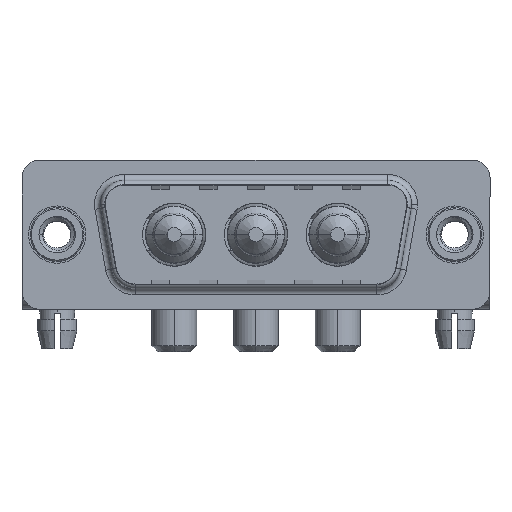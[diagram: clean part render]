
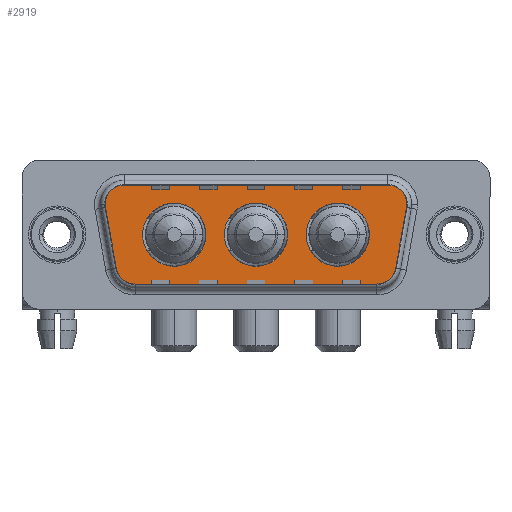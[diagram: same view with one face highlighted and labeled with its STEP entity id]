
A CAD part, top view. The second image highlights one B-rep face of the part: STEP entity #2919.
In plain terms, the highlighted planar face has unit normal (0, 0, 1).
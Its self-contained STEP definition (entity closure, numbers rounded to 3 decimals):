
#62 = CIRCLE ( 'NONE', #9373, 2. ) ;
#112 = DIRECTION ( 'NONE',  ( 0., 0., 1. ) ) ;
#334 = AXIS2_PLACEMENT_3D ( 'NONE', #9190, #4175, #4257 ) ;
#494 = VERTEX_POINT ( 'NONE', #16074 ) ;
#669 = ORIENTED_EDGE ( 'NONE', *, *, #7962, .T. ) ;
#758 = FACE_OUTER_BOUND ( 'NONE', #4294, .T. ) ;
#973 = VERTEX_POINT ( 'NONE', #8131 ) ;
#975 = DIRECTION ( 'NONE',  ( 0.174, -0.985, 0. ) ) ;
#1321 = CARTESIAN_POINT ( 'NONE',  ( 4.464, -3.247, 0. ) ) ;
#1376 = CIRCLE ( 'NONE', #2183, 2. ) ;
#1502 = EDGE_LOOP ( 'NONE', ( #6239, #13874 ) ) ;
#2003 = ORIENTED_EDGE ( 'NONE', *, *, #2544, .T. ) ;
#2026 = DIRECTION ( 'NONE',  ( 0., 0., 1. ) ) ;
#2038 = EDGE_CURVE ( 'NONE', #14971, #13674, #3644, .T. ) ;
#2063 = DIRECTION ( 'NONE',  ( 0., 0., 1. ) ) ;
#2183 = AXIS2_PLACEMENT_3D ( 'NONE', #11516, #112, #14067 ) ;
#2236 = ORIENTED_EDGE ( 'NONE', *, *, #15955, .T. ) ;
#2244 = CARTESIAN_POINT ( 'NONE',  ( 19.3, 0., 0. ) ) ;
#2288 = DIRECTION ( 'NONE',  ( -1., 0., 0. ) ) ;
#2383 = CIRCLE ( 'NONE', #10091, 2. ) ;
#2413 = CARTESIAN_POINT ( 'NONE',  ( 3.441, 2.553, 0. ) ) ;
#2451 = DIRECTION ( 'NONE',  ( 0., 0., 1. ) ) ;
#2472 = VERTEX_POINT ( 'NONE', #14736 ) ;
#2508 = CARTESIAN_POINT ( 'NONE',  ( 27.889, 4.9, 0. ) ) ;
#2544 = EDGE_CURVE ( 'NONE', #7589, #12192, #7376, .T. ) ;
#2668 = AXIS2_PLACEMENT_3D ( 'NONE', #5523, #10586, #3020 ) ;
#2671 = CARTESIAN_POINT ( 'NONE',  ( 6.434, -4.9, 0. ) ) ;
#2919 = ADVANCED_FACE ( 'NONE', ( #9772, #12248, #7093, #758 ), #3181, .T. ) ;
#3020 = DIRECTION ( 'NONE',  ( 1., 0., 0. ) ) ;
#3071 = ORIENTED_EDGE ( 'NONE', *, *, #7793, .T. ) ;
#3181 = PLANE ( 'NONE',  #11221 ) ;
#3267 = DIRECTION ( 'NONE',  ( 0., 0., 1. ) ) ;
#3330 = CARTESIAN_POINT ( 'NONE',  ( 7.15, 0., 0. ) ) ;
#3361 = CARTESIAN_POINT ( 'NONE',  ( 26.866, -4.9, 0. ) ) ;
#3372 = DIRECTION ( 'NONE',  ( -1., 0., 0. ) ) ;
#3630 = EDGE_CURVE ( 'NONE', #5560, #13367, #10240, .T. ) ;
#3644 = LINE ( 'NONE', #16088, #15944 ) ;
#3901 = CARTESIAN_POINT ( 'NONE',  ( 16.65, 0., 0. ) ) ;
#3973 = CIRCLE ( 'NONE', #14322, 2.65 ) ;
#4175 = DIRECTION ( 'NONE',  ( 0., 0., 1. ) ) ;
#4257 = DIRECTION ( 'NONE',  ( 1., 0., 0. ) ) ;
#4294 = EDGE_LOOP ( 'NONE', ( #5574, #669, #2236, #9229, #2003, #10066, #11195, #3071, #12345 ) ) ;
#4396 = CARTESIAN_POINT ( 'NONE',  ( 6.434, -2.9, 0. ) ) ;
#4527 = CIRCLE ( 'NONE', #9333, 2. ) ;
#4597 = CARTESIAN_POINT ( 'NONE',  ( 26.866, -2.9, 0. ) ) ;
#4657 = VERTEX_POINT ( 'NONE', #12388 ) ;
#4755 = CIRCLE ( 'NONE', #11416, 2.65 ) ;
#4865 = EDGE_CURVE ( 'NONE', #13472, #2472, #13199, .T. ) ;
#5523 = CARTESIAN_POINT ( 'NONE',  ( 16.65, 0., 0. ) ) ;
#5560 = VERTEX_POINT ( 'NONE', #10614 ) ;
#5574 = ORIENTED_EDGE ( 'NONE', *, *, #9288, .T. ) ;
#5813 = DIRECTION ( 'NONE',  ( 0., 0., 1. ) ) ;
#5927 = ORIENTED_EDGE ( 'NONE', *, *, #12511, .F. ) ;
#6073 = LINE ( 'NONE', #7316, #9551 ) ;
#6239 = ORIENTED_EDGE ( 'NONE', *, *, #7839, .F. ) ;
#6382 = DIRECTION ( 'NONE',  ( 0.174, 0.985, 0. ) ) ;
#6457 = CIRCLE ( 'NONE', #334, 2.65 ) ;
#6818 = ORIENTED_EDGE ( 'NONE', *, *, #16367, .F. ) ;
#6961 = VERTEX_POINT ( 'NONE', #14890 ) ;
#6987 = DIRECTION ( 'NONE',  ( 1., 0., 0. ) ) ;
#7093 = FACE_BOUND ( 'NONE', #1502, .T. ) ;
#7098 = DIRECTION ( 'NONE',  ( 0., 0., 1. ) ) ;
#7143 = DIRECTION ( 'NONE',  ( -1., 0., 0. ) ) ;
#7196 = DIRECTION ( 'NONE',  ( 0., 0., 1. ) ) ;
#7282 = CARTESIAN_POINT ( 'NONE',  ( 26.866, -2.9, 0. ) ) ;
#7316 = CARTESIAN_POINT ( 'NONE',  ( 29.859, 2.553, 0. ) ) ;
#7376 = LINE ( 'NONE', #16160, #10085 ) ;
#7571 = CARTESIAN_POINT ( 'NONE',  ( 28.836, -3.247, 0. ) ) ;
#7579 = DIRECTION ( 'NONE',  ( 0., 0., 1. ) ) ;
#7589 = VERTEX_POINT ( 'NONE', #2508 ) ;
#7793 = EDGE_CURVE ( 'NONE', #13674, #5560, #16162, .T. ) ;
#7839 = EDGE_CURVE ( 'NONE', #494, #14833, #8766, .T. ) ;
#7939 = EDGE_CURVE ( 'NONE', #6961, #10561, #4755, .T. ) ;
#7962 = EDGE_CURVE ( 'NONE', #13678, #4657, #6073, .T. ) ;
#7992 = CIRCLE ( 'NONE', #2668, 2.65 ) ;
#8085 = CARTESIAN_POINT ( 'NONE',  ( 9.8, 0., 0. ) ) ;
#8131 = CARTESIAN_POINT ( 'NONE',  ( 29.889, 2.9, 0. ) ) ;
#8205 = EDGE_CURVE ( 'NONE', #14833, #494, #3973, .T. ) ;
#8539 = EDGE_LOOP ( 'NONE', ( #15454, #6818 ) ) ;
#8766 = CIRCLE ( 'NONE', #10340, 2.65 ) ;
#8877 = ORIENTED_EDGE ( 'NONE', *, *, #7939, .F. ) ;
#9190 = CARTESIAN_POINT ( 'NONE',  ( 23.5, 0., 0. ) ) ;
#9229 = ORIENTED_EDGE ( 'NONE', *, *, #12209, .T. ) ;
#9256 = AXIS2_PLACEMENT_3D ( 'NONE', #3901, #7579, #15112 ) ;
#9288 = EDGE_CURVE ( 'NONE', #13367, #13678, #4527, .T. ) ;
#9333 = AXIS2_PLACEMENT_3D ( 'NONE', #7282, #7196, #9531 ) ;
#9373 = AXIS2_PLACEMENT_3D ( 'NONE', #10108, #2451, #12837 ) ;
#9531 = DIRECTION ( 'NONE',  ( 1., 0., 0. ) ) ;
#9551 = VECTOR ( 'NONE', #6382, 1000. ) ;
#9772 = FACE_BOUND ( 'NONE', #8539, .T. ) ;
#10066 = ORIENTED_EDGE ( 'NONE', *, *, #12267, .T. ) ;
#10085 = VECTOR ( 'NONE', #3372, 1000. ) ;
#10091 = AXIS2_PLACEMENT_3D ( 'NONE', #12099, #2026, #2288 ) ;
#10108 = CARTESIAN_POINT ( 'NONE',  ( 27.889, 2.9, 0. ) ) ;
#10240 = LINE ( 'NONE', #2671, #12656 ) ;
#10340 = AXIS2_PLACEMENT_3D ( 'NONE', #8085, #5813, #6987 ) ;
#10561 = VERTEX_POINT ( 'NONE', #11899 ) ;
#10586 = DIRECTION ( 'NONE',  ( 0., 0., 1. ) ) ;
#10614 = CARTESIAN_POINT ( 'NONE',  ( 6.434, -4.9, 0. ) ) ;
#11195 = ORIENTED_EDGE ( 'NONE', *, *, #2038, .T. ) ;
#11221 = AXIS2_PLACEMENT_3D ( 'NONE', #4597, #3267, #15960 ) ;
#11322 = DIRECTION ( 'NONE',  ( 1., 0., 0. ) ) ;
#11416 = AXIS2_PLACEMENT_3D ( 'NONE', #14844, #16093, #14758 ) ;
#11516 = CARTESIAN_POINT ( 'NONE',  ( 5.411, 2.9, 0. ) ) ;
#11899 = CARTESIAN_POINT ( 'NONE',  ( 26.15, 0., 0. ) ) ;
#12099 = CARTESIAN_POINT ( 'NONE',  ( 27.889, 2.9, 0. ) ) ;
#12167 = DIRECTION ( 'NONE',  ( 1., 0., 0. ) ) ;
#12192 = VERTEX_POINT ( 'NONE', #12753 ) ;
#12209 = EDGE_CURVE ( 'NONE', #973, #7589, #62, .T. ) ;
#12248 = FACE_BOUND ( 'NONE', #13264, .T. ) ;
#12267 = EDGE_CURVE ( 'NONE', #12192, #14971, #1376, .T. ) ;
#12345 = ORIENTED_EDGE ( 'NONE', *, *, #3630, .T. ) ;
#12388 = CARTESIAN_POINT ( 'NONE',  ( 29.859, 2.553, 0. ) ) ;
#12511 = EDGE_CURVE ( 'NONE', #10561, #6961, #6457, .T. ) ;
#12656 = VECTOR ( 'NONE', #11322, 1000. ) ;
#12728 = AXIS2_PLACEMENT_3D ( 'NONE', #4396, #2063, #7143 ) ;
#12753 = CARTESIAN_POINT ( 'NONE',  ( 5.411, 4.9, 0. ) ) ;
#12837 = DIRECTION ( 'NONE',  ( -1., 0., 0. ) ) ;
#13199 = CIRCLE ( 'NONE', #9256, 2.65 ) ;
#13264 = EDGE_LOOP ( 'NONE', ( #5927, #8877 ) ) ;
#13367 = VERTEX_POINT ( 'NONE', #3361 ) ;
#13472 = VERTEX_POINT ( 'NONE', #2244 ) ;
#13674 = VERTEX_POINT ( 'NONE', #1321 ) ;
#13678 = VERTEX_POINT ( 'NONE', #7571 ) ;
#13874 = ORIENTED_EDGE ( 'NONE', *, *, #8205, .F. ) ;
#14067 = DIRECTION ( 'NONE',  ( 1., 0., 0. ) ) ;
#14322 = AXIS2_PLACEMENT_3D ( 'NONE', #14716, #7098, #12167 ) ;
#14716 = CARTESIAN_POINT ( 'NONE',  ( 9.8, 0., 0. ) ) ;
#14736 = CARTESIAN_POINT ( 'NONE',  ( 14., 0., 0. ) ) ;
#14758 = DIRECTION ( 'NONE',  ( 1., 0., 0. ) ) ;
#14833 = VERTEX_POINT ( 'NONE', #3330 ) ;
#14844 = CARTESIAN_POINT ( 'NONE',  ( 23.5, 0., 0. ) ) ;
#14890 = CARTESIAN_POINT ( 'NONE',  ( 20.85, 0., 0. ) ) ;
#14971 = VERTEX_POINT ( 'NONE', #2413 ) ;
#15112 = DIRECTION ( 'NONE',  ( 1., 0., 0. ) ) ;
#15454 = ORIENTED_EDGE ( 'NONE', *, *, #4865, .F. ) ;
#15944 = VECTOR ( 'NONE', #975, 1000. ) ;
#15955 = EDGE_CURVE ( 'NONE', #4657, #973, #2383, .T. ) ;
#15960 = DIRECTION ( 'NONE',  ( 1., 0., 0. ) ) ;
#16074 = CARTESIAN_POINT ( 'NONE',  ( 12.45, 0., 0. ) ) ;
#16088 = CARTESIAN_POINT ( 'NONE',  ( 3.441, 2.553, 0. ) ) ;
#16093 = DIRECTION ( 'NONE',  ( 0., 0., 1. ) ) ;
#16160 = CARTESIAN_POINT ( 'NONE',  ( 5.411, 4.9, 0. ) ) ;
#16162 = CIRCLE ( 'NONE', #12728, 2. ) ;
#16367 = EDGE_CURVE ( 'NONE', #2472, #13472, #7992, .T. ) ;
